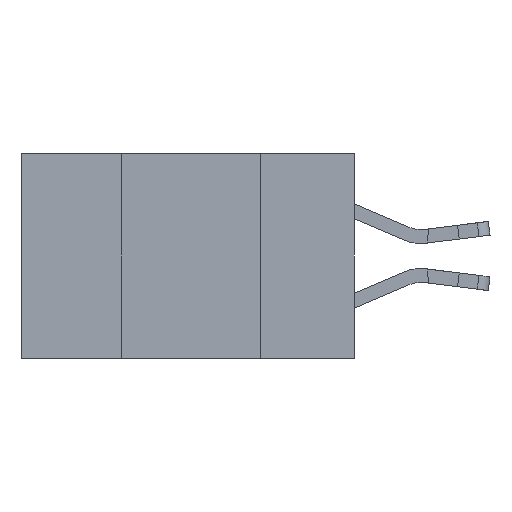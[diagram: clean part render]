
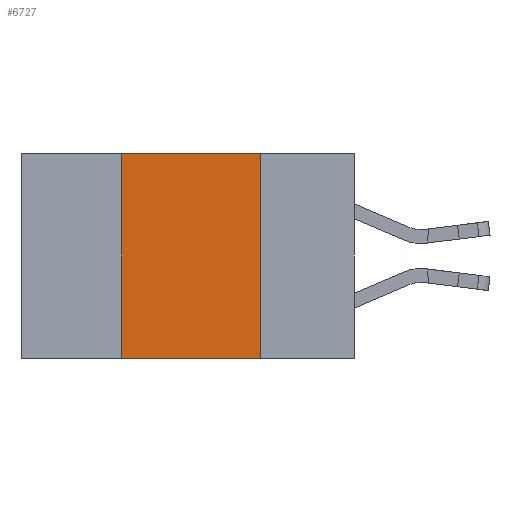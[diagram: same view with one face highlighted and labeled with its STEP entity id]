
A CAD part, left-side view. The second image highlights one B-rep face of the part: STEP entity #6727.
In plain terms, the highlighted planar face has unit normal (-1, 0, 0).
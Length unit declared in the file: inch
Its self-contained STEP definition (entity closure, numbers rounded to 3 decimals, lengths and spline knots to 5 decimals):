
#311 = VERTEX_POINT ( 'NONE', #3234 ) ;
#531 = FACE_OUTER_BOUND ( 'NONE', #3647, .T. ) ;
#621 = ORIENTED_EDGE ( 'NONE', *, *, #1619, .F. ) ;
#635 = DIRECTION ( 'NONE',  ( 0., 0., 1. ) ) ;
#1125 = CARTESIAN_POINT ( 'NONE',  ( 0., 0.6, -0.37 ) ) ;
#1242 = CARTESIAN_POINT ( 'NONE',  ( 0., 0.42, -0.37 ) ) ;
#1607 = DIRECTION ( 'NONE',  ( 0., -1., 0. ) ) ;
#1619 = EDGE_CURVE ( 'NONE', #6757, #311, #6976, .T. ) ;
#2267 = DIRECTION ( 'NONE',  ( 0., 0., -1. ) ) ;
#2380 = CARTESIAN_POINT ( 'NONE',  ( 0., 0.42, -0.37 ) ) ;
#3063 = DIRECTION ( 'NONE',  ( 0., -1., 0. ) ) ;
#3175 = VECTOR ( 'NONE', #8673, 39.37008 ) ;
#3234 = CARTESIAN_POINT ( 'NONE',  ( 0., 0.17, -0.37 ) ) ;
#3540 = CARTESIAN_POINT ( 'NONE',  ( 0., 0.17, -0.37 ) ) ;
#3609 = EDGE_CURVE ( 'NONE', #6179, #8232, #10417, .T. ) ;
#3647 = EDGE_LOOP ( 'NONE', ( #621, #6348, #6097, #9203 ) ) ;
#4101 = CARTESIAN_POINT ( 'NONE',  ( 0., 0.6, 0. ) ) ;
#4432 = EDGE_CURVE ( 'NONE', #8232, #6757, #7806, .T. ) ;
#4656 = EDGE_CURVE ( 'NONE', #6179, #311, #10094, .T. ) ;
#6097 = ORIENTED_EDGE ( 'NONE', *, *, #3609, .F. ) ;
#6179 = VERTEX_POINT ( 'NONE', #1242 ) ;
#6348 = ORIENTED_EDGE ( 'NONE', *, *, #4432, .F. ) ;
#6416 = VECTOR ( 'NONE', #1607, 39.37008 ) ;
#6727 = ADVANCED_FACE ( 'NONE', ( #531 ), #6896, .F. ) ;
#6757 = VERTEX_POINT ( 'NONE', #7660 ) ;
#6896 = PLANE ( 'NONE',  #10478 ) ;
#6976 = LINE ( 'NONE', #3540, #3175 ) ;
#7402 = VECTOR ( 'NONE', #3063, 39.37008 ) ;
#7660 = CARTESIAN_POINT ( 'NONE',  ( 0., 0.17, 0. ) ) ;
#7806 = LINE ( 'NONE', #10626, #6416 ) ;
#8232 = VERTEX_POINT ( 'NONE', #10898 ) ;
#8673 = DIRECTION ( 'NONE',  ( 0., 0., -1. ) ) ;
#9203 = ORIENTED_EDGE ( 'NONE', *, *, #4656, .T. ) ;
#10094 = LINE ( 'NONE', #1125, #7402 ) ;
#10366 = VECTOR ( 'NONE', #635, 39.37008 ) ;
#10373 = DIRECTION ( 'NONE',  ( 1., 0., 0. ) ) ;
#10417 = LINE ( 'NONE', #2380, #10366 ) ;
#10478 = AXIS2_PLACEMENT_3D ( 'NONE', #4101, #10373, #2267 ) ;
#10626 = CARTESIAN_POINT ( 'NONE',  ( 0., 0.6, 0. ) ) ;
#10898 = CARTESIAN_POINT ( 'NONE',  ( 0., 0.42, 0. ) ) ;
